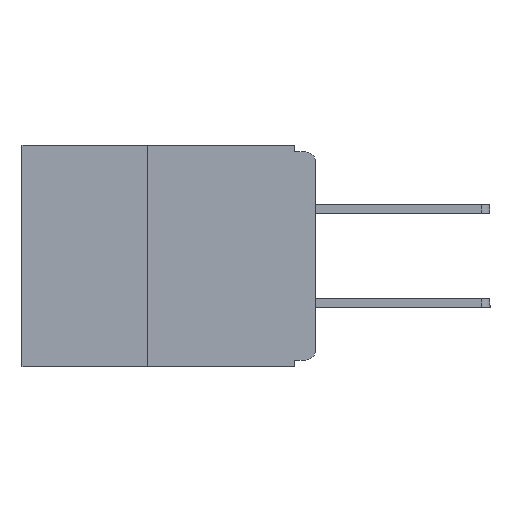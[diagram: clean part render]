
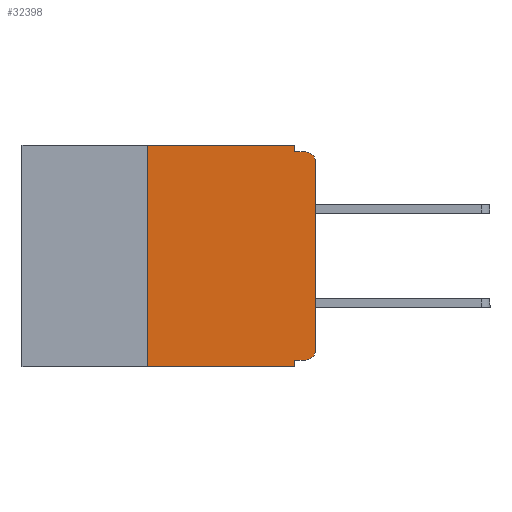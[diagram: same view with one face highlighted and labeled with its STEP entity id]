
A CAD part, left-side view. The second image highlights one B-rep face of the part: STEP entity #32398.
In plain terms, the highlighted planar face has unit normal (-1, 0, 0).
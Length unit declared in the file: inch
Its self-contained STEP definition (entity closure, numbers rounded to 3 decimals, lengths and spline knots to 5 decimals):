
#228 = ORIENTED_EDGE ( 'NONE', *, *, #32943, .F. ) ;
#297 = DIRECTION ( 'NONE',  ( 0., 0., -1. ) ) ;
#339 = CARTESIAN_POINT ( 'NONE',  ( 0., 0.015, -0.025 ) ) ;
#576 = EDGE_CURVE ( 'NONE', #28009, #17329, #9801, .T. ) ;
#950 = CARTESIAN_POINT ( 'NONE',  ( 0., 0.25, -0.33 ) ) ;
#1398 = CARTESIAN_POINT ( 'NONE',  ( 0., 0., -0.025 ) ) ;
#2528 = CARTESIAN_POINT ( 'NONE',  ( 0., 0.437, -0.33 ) ) ;
#2908 = DIRECTION ( 'NONE',  ( 0., 0., -1. ) ) ;
#3528 = DIRECTION ( 'NONE',  ( 0., 0., 1. ) ) ;
#3615 = FACE_OUTER_BOUND ( 'NONE', #6186, .T. ) ;
#3872 = ORIENTED_EDGE ( 'NONE', *, *, #21078, .F. ) ;
#4457 = VERTEX_POINT ( 'NONE', #15131 ) ;
#4495 = VECTOR ( 'NONE', #25922, 39.37008 ) ;
#4868 = CARTESIAN_POINT ( 'NONE',  ( 0., 0.437, 0. ) ) ;
#5575 = LINE ( 'NONE', #950, #30988 ) ;
#5872 = ORIENTED_EDGE ( 'NONE', *, *, #29098, .T. ) ;
#6186 = EDGE_LOOP ( 'NONE', ( #22984, #5872, #8275, #228, #15036, #3872, #11802, #25386, #21769, #15798 ) ) ;
#7700 = CARTESIAN_POINT ( 'NONE',  ( 0., 0.015, -0.01 ) ) ;
#8017 = VERTEX_POINT ( 'NONE', #7700 ) ;
#8180 = LINE ( 'NONE', #4868, #28457 ) ;
#8275 = ORIENTED_EDGE ( 'NONE', *, *, #25516, .F. ) ;
#9801 = LINE ( 'NONE', #2528, #29300 ) ;
#10257 = VERTEX_POINT ( 'NONE', #27071 ) ;
#10428 = LINE ( 'NONE', #21938, #23197 ) ;
#10442 = DIRECTION ( 'NONE',  ( 0., 1., 0. ) ) ;
#10790 = CARTESIAN_POINT ( 'NONE',  ( 0., 0.25, -0.33 ) ) ;
#11565 = CARTESIAN_POINT ( 'NONE',  ( 0., 0.031, -0.01 ) ) ;
#11802 = ORIENTED_EDGE ( 'NONE', *, *, #576, .T. ) ;
#12643 = DIRECTION ( 'NONE',  ( 0., 0., -1. ) ) ;
#12802 = VERTEX_POINT ( 'NONE', #17148 ) ;
#13336 = VERTEX_POINT ( 'NONE', #11565 ) ;
#13363 = VECTOR ( 'NONE', #24933, 39.37008 ) ;
#15036 = ORIENTED_EDGE ( 'NONE', *, *, #30733, .F. ) ;
#15068 = PLANE ( 'NONE',  #18040 ) ;
#15131 = CARTESIAN_POINT ( 'NONE',  ( 0., 0.031, 0. ) ) ;
#15368 = DIRECTION ( 'NONE',  ( 0., 0., -1. ) ) ;
#15558 = CARTESIAN_POINT ( 'NONE',  ( 0., 0., -0.32 ) ) ;
#15590 = DIRECTION ( 'NONE',  ( -1., 0., 0. ) ) ;
#15798 = ORIENTED_EDGE ( 'NONE', *, *, #29709, .T. ) ;
#17148 = CARTESIAN_POINT ( 'NONE',  ( 0., 0.015, -0.32 ) ) ;
#17329 = VERTEX_POINT ( 'NONE', #28189 ) ;
#18040 = AXIS2_PLACEMENT_3D ( 'NONE', #22768, #27876, #12643 ) ;
#18162 = DIRECTION ( 'NONE',  ( -1., 0., 0. ) ) ;
#18183 = CARTESIAN_POINT ( 'NONE',  ( 0., 0.031, -0.33 ) ) ;
#18479 = CARTESIAN_POINT ( 'NONE',  ( 0., 0., -0.305 ) ) ;
#18943 = CIRCLE ( 'NONE', #22740, 0.015 ) ;
#20450 = CARTESIAN_POINT ( 'NONE',  ( 0., 0.031, 0. ) ) ;
#20694 = LINE ( 'NONE', #20450, #25935 ) ;
#21078 = EDGE_CURVE ( 'NONE', #28009, #10257, #5575, .T. ) ;
#21769 = ORIENTED_EDGE ( 'NONE', *, *, #28453, .F. ) ;
#21938 = CARTESIAN_POINT ( 'NONE',  ( 0., 0., 0. ) ) ;
#22345 = CARTESIAN_POINT ( 'NONE',  ( 0., 0., -0.01 ) ) ;
#22691 = DIRECTION ( 'NONE',  ( 0., -1., 0. ) ) ;
#22740 = AXIS2_PLACEMENT_3D ( 'NONE', #30789, #15590, #297 ) ;
#22768 = CARTESIAN_POINT ( 'NONE',  ( 0., 0.437, 0. ) ) ;
#22874 = VERTEX_POINT ( 'NONE', #1398 ) ;
#22984 = ORIENTED_EDGE ( 'NONE', *, *, #28258, .T. ) ;
#23197 = VECTOR ( 'NONE', #24533, 39.37008 ) ;
#24017 = VERTEX_POINT ( 'NONE', #26218 ) ;
#24024 = AXIS2_PLACEMENT_3D ( 'NONE', #339, #18162, #2908 ) ;
#24533 = DIRECTION ( 'NONE',  ( 0., 0., 1. ) ) ;
#24933 = DIRECTION ( 'NONE',  ( 0., -1., 0. ) ) ;
#25386 = ORIENTED_EDGE ( 'NONE', *, *, #31904, .F. ) ;
#25516 = EDGE_CURVE ( 'NONE', #13336, #8017, #27723, .T. ) ;
#25594 = VERTEX_POINT ( 'NONE', #18479 ) ;
#25922 = DIRECTION ( 'NONE',  ( 0., 0., -1. ) ) ;
#25935 = VECTOR ( 'NONE', #15368, 39.37008 ) ;
#25982 = LINE ( 'NONE', #15558, #30290 ) ;
#26218 = CARTESIAN_POINT ( 'NONE',  ( 0., 0.031, -0.32 ) ) ;
#27071 = CARTESIAN_POINT ( 'NONE',  ( 0., 0.25, 0. ) ) ;
#27723 = LINE ( 'NONE', #22345, #13363 ) ;
#27876 = DIRECTION ( 'NONE',  ( 1., 0., 0. ) ) ;
#28009 = VERTEX_POINT ( 'NONE', #10790 ) ;
#28189 = CARTESIAN_POINT ( 'NONE',  ( 0., 0.031, -0.33 ) ) ;
#28258 = EDGE_CURVE ( 'NONE', #25594, #22874, #10428, .T. ) ;
#28313 = DIRECTION ( 'NONE',  ( 0., -1., 0. ) ) ;
#28453 = EDGE_CURVE ( 'NONE', #12802, #24017, #25982, .T. ) ;
#28457 = VECTOR ( 'NONE', #22691, 39.37008 ) ;
#29098 = EDGE_CURVE ( 'NONE', #22874, #8017, #31419, .T. ) ;
#29300 = VECTOR ( 'NONE', #28313, 39.37008 ) ;
#29709 = EDGE_CURVE ( 'NONE', #12802, #25594, #18943, .T. ) ;
#30290 = VECTOR ( 'NONE', #10442, 39.37008 ) ;
#30733 = EDGE_CURVE ( 'NONE', #10257, #4457, #8180, .T. ) ;
#30789 = CARTESIAN_POINT ( 'NONE',  ( 0., 0.015, -0.305 ) ) ;
#30988 = VECTOR ( 'NONE', #3528, 39.37008 ) ;
#31419 = CIRCLE ( 'NONE', #24024, 0.015 ) ;
#31493 = LINE ( 'NONE', #18183, #4495 ) ;
#31904 = EDGE_CURVE ( 'NONE', #24017, #17329, #31493, .T. ) ;
#32398 = ADVANCED_FACE ( 'NONE', ( #3615 ), #15068, .F. ) ;
#32943 = EDGE_CURVE ( 'NONE', #4457, #13336, #20694, .T. ) ;
